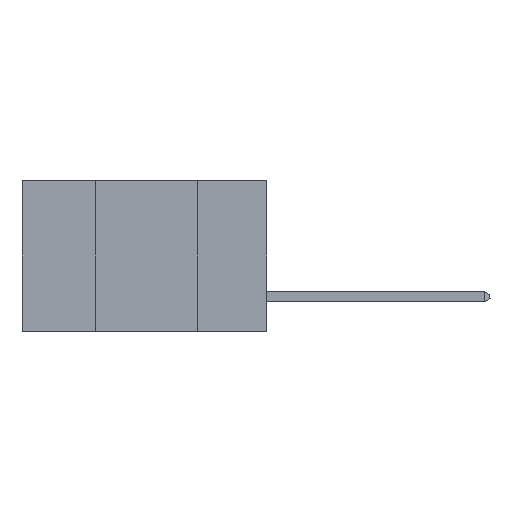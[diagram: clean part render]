
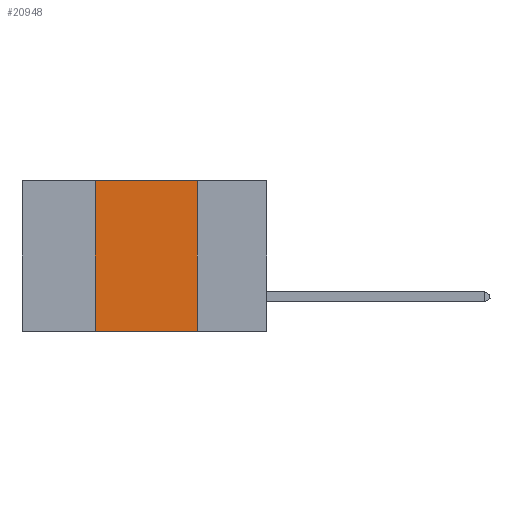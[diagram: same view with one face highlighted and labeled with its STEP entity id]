
A CAD part, left-side view. The second image highlights one B-rep face of the part: STEP entity #20948.
In plain terms, the highlighted planar face has unit normal (-1, 0, 0).
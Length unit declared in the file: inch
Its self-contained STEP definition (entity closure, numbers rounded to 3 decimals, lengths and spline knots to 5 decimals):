
#307 = EDGE_CURVE ( 'NONE', #23764, #12680, #4708, .T. ) ;
#1475 = PLANE ( 'NONE',  #15470 ) ;
#1608 = CARTESIAN_POINT ( 'NONE',  ( 0., 0.6, 0. ) ) ;
#2599 = DIRECTION ( 'NONE',  ( 1., 0., 0. ) ) ;
#3228 = DIRECTION ( 'NONE',  ( 0., 0., -1. ) ) ;
#3375 = VERTEX_POINT ( 'NONE', #38320 ) ;
#3588 = EDGE_CURVE ( 'NONE', #3375, #38515, #32130, .T. ) ;
#4127 = ORIENTED_EDGE ( 'NONE', *, *, #3588, .F. ) ;
#4629 = DIRECTION ( 'NONE',  ( 0., -1., 0. ) ) ;
#4708 = LINE ( 'NONE', #32550, #10661 ) ;
#4961 = VECTOR ( 'NONE', #31461, 39.37008 ) ;
#5989 = CARTESIAN_POINT ( 'NONE',  ( 0., 0.6, 0. ) ) ;
#8876 = EDGE_CURVE ( 'NONE', #38515, #12680, #36665, .T. ) ;
#10661 = VECTOR ( 'NONE', #4629, 39.37008 ) ;
#11703 = DIRECTION ( 'NONE',  ( 0., 0., 1. ) ) ;
#12494 = ORIENTED_EDGE ( 'NONE', *, *, #36659, .F. ) ;
#12680 = VERTEX_POINT ( 'NONE', #18388 ) ;
#13145 = CARTESIAN_POINT ( 'NONE',  ( 0., 0.17, 0. ) ) ;
#13204 = EDGE_LOOP ( 'NONE', ( #14007, #4127, #12494, #30846 ) ) ;
#14007 = ORIENTED_EDGE ( 'NONE', *, *, #8876, .F. ) ;
#15470 = AXIS2_PLACEMENT_3D ( 'NONE', #1608, #2599, #24896 ) ;
#17217 = CARTESIAN_POINT ( 'NONE',  ( 0., 0.42, 0. ) ) ;
#18388 = CARTESIAN_POINT ( 'NONE',  ( 0., 0.17, -0.37 ) ) ;
#20948 = ADVANCED_FACE ( 'NONE', ( #27461 ), #1475, .F. ) ;
#22264 = LINE ( 'NONE', #17217, #27292 ) ;
#23764 = VERTEX_POINT ( 'NONE', #28959 ) ;
#24896 = DIRECTION ( 'NONE',  ( 0., 0., -1. ) ) ;
#27292 = VECTOR ( 'NONE', #11703, 39.37008 ) ;
#27461 = FACE_OUTER_BOUND ( 'NONE', #13204, .T. ) ;
#28959 = CARTESIAN_POINT ( 'NONE',  ( 0., 0.42, -0.37 ) ) ;
#29606 = VECTOR ( 'NONE', #3228, 39.37008 ) ;
#30846 = ORIENTED_EDGE ( 'NONE', *, *, #307, .T. ) ;
#31461 = DIRECTION ( 'NONE',  ( 0., -1., 0. ) ) ;
#32130 = LINE ( 'NONE', #5989, #4961 ) ;
#32550 = CARTESIAN_POINT ( 'NONE',  ( 0., 0.6, -0.37 ) ) ;
#36659 = EDGE_CURVE ( 'NONE', #23764, #3375, #22264, .T. ) ;
#36665 = LINE ( 'NONE', #13145, #29606 ) ;
#37220 = CARTESIAN_POINT ( 'NONE',  ( 0., 0.17, 0. ) ) ;
#38320 = CARTESIAN_POINT ( 'NONE',  ( 0., 0.42, 0. ) ) ;
#38515 = VERTEX_POINT ( 'NONE', #37220 ) ;
